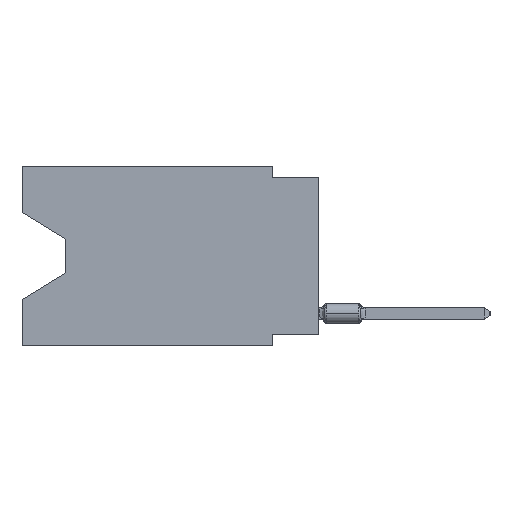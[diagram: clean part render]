
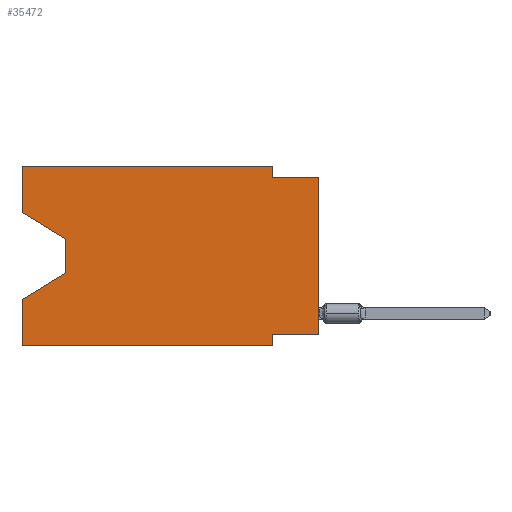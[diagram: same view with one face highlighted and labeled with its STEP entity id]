
A CAD part, left-side view. The second image highlights one B-rep face of the part: STEP entity #35472.
In plain terms, the highlighted planar face has unit normal (-1, 0, 0).
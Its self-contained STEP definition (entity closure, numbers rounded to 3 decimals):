
#967 = VERTEX_POINT ( 'NONE', #29241 ) ;
#978 = LINE ( 'NONE', #5575, #1717 ) ;
#1210 = CARTESIAN_POINT ( 'NONE',  ( 0., 0., -0.635 ) ) ;
#1267 = DIRECTION ( 'NONE',  ( 0., 0., 1. ) ) ;
#1576 = DIRECTION ( 'NONE',  ( 0., 0., 1. ) ) ;
#1717 = VECTOR ( 'NONE', #1576, 1000. ) ;
#2077 = VERTEX_POINT ( 'NONE', #21697 ) ;
#2115 = LINE ( 'NONE', #16244, #34366 ) ;
#3114 = EDGE_CURVE ( 'NONE', #31184, #11904, #978, .T. ) ;
#3126 = CARTESIAN_POINT ( 'NONE',  ( 0., 0., 0. ) ) ;
#5131 = EDGE_CURVE ( 'NONE', #29880, #53649, #2115, .T. ) ;
#5323 = EDGE_LOOP ( 'NONE', ( #9318, #32974, #53867, #51299, #5969, #42770, #48127, #58527, #47879, #10838, #58053, #54264 ) ) ;
#5575 = CARTESIAN_POINT ( 'NONE',  ( 0., 16.383, 0. ) ) ;
#5668 = VECTOR ( 'NONE', #20472, 1000. ) ;
#5870 = CARTESIAN_POINT ( 'NONE',  ( 0., 16.383, 0. ) ) ;
#5969 = ORIENTED_EDGE ( 'NONE', *, *, #59230, .T. ) ;
#6112 = PLANE ( 'NONE',  #14296 ) ;
#6342 = LINE ( 'NONE', #15268, #5668 ) ;
#6634 = CARTESIAN_POINT ( 'NONE',  ( 0., 16.383, -2.546 ) ) ;
#6934 = LINE ( 'NONE', #19030, #54746 ) ;
#7481 = LINE ( 'NONE', #58170, #37484 ) ;
#7900 = EDGE_CURVE ( 'NONE', #38194, #13895, #7481, .T. ) ;
#8309 = CARTESIAN_POINT ( 'NONE',  ( 0., 16.383, 0. ) ) ;
#9318 = ORIENTED_EDGE ( 'NONE', *, *, #32489, .T. ) ;
#9823 = DIRECTION ( 'NONE',  ( 0., 0., -1. ) ) ;
#10111 = DIRECTION ( 'NONE',  ( 0., 0., -1. ) ) ;
#10654 = LINE ( 'NONE', #14659, #21511 ) ;
#10771 = LINE ( 'NONE', #20596, #28127 ) ;
#10838 = ORIENTED_EDGE ( 'NONE', *, *, #7900, .F. ) ;
#11307 = CARTESIAN_POINT ( 'NONE',  ( 0., 13.97, -5.893 ) ) ;
#11727 = EDGE_CURVE ( 'NONE', #967, #2077, #53460, .T. ) ;
#11904 = VERTEX_POINT ( 'NONE', #8309 ) ;
#13895 = VERTEX_POINT ( 'NONE', #43415 ) ;
#14072 = VECTOR ( 'NONE', #20836, 1000. ) ;
#14296 = AXIS2_PLACEMENT_3D ( 'NONE', #24871, #57719, #9823 ) ;
#14659 = CARTESIAN_POINT ( 'NONE',  ( 0., 0., -9.271 ) ) ;
#15268 = CARTESIAN_POINT ( 'NONE',  ( 0., 16.383, 0. ) ) ;
#15713 = CARTESIAN_POINT ( 'NONE',  ( 0., 2.54, -9.906 ) ) ;
#15995 = DIRECTION ( 'NONE',  ( 0., -1., 0. ) ) ;
#16244 = CARTESIAN_POINT ( 'NONE',  ( 0., 2.54, -9.906 ) ) ;
#16991 = LINE ( 'NONE', #21292, #18967 ) ;
#18967 = VECTOR ( 'NONE', #20376, 1000. ) ;
#19030 = CARTESIAN_POINT ( 'NONE',  ( 0., 13.97, -4.013 ) ) ;
#19507 = DIRECTION ( 'NONE',  ( 0., -1., 0. ) ) ;
#20376 = DIRECTION ( 'NONE',  ( 0., -0.855, -0.519 ) ) ;
#20472 = DIRECTION ( 'NONE',  ( 0., -1., 0. ) ) ;
#20596 = CARTESIAN_POINT ( 'NONE',  ( 0., 0., -0.635 ) ) ;
#20694 = DIRECTION ( 'NONE',  ( 0., 0., -1. ) ) ;
#20836 = DIRECTION ( 'NONE',  ( 0., 0.855, -0.519 ) ) ;
#20848 = DIRECTION ( 'NONE',  ( 0., 0., -1. ) ) ;
#21292 = CARTESIAN_POINT ( 'NONE',  ( 0., 16.383, -2.546 ) ) ;
#21511 = VECTOR ( 'NONE', #52436, 1000. ) ;
#21697 = CARTESIAN_POINT ( 'NONE',  ( 0., 16.383, -7.36 ) ) ;
#24871 = CARTESIAN_POINT ( 'NONE',  ( 0., 16.383, 0. ) ) ;
#25377 = CARTESIAN_POINT ( 'NONE',  ( 0., 2.54, -9.271 ) ) ;
#25723 = EDGE_CURVE ( 'NONE', #29432, #28521, #31078, .T. ) ;
#27643 = CARTESIAN_POINT ( 'NONE',  ( 0., 2.54, 0. ) ) ;
#28127 = VECTOR ( 'NONE', #15995, 1000. ) ;
#28521 = VERTEX_POINT ( 'NONE', #1210 ) ;
#29241 = CARTESIAN_POINT ( 'NONE',  ( 0., 16.383, -9.906 ) ) ;
#29271 = VECTOR ( 'NONE', #1267, 1000. ) ;
#29432 = VERTEX_POINT ( 'NONE', #54472 ) ;
#29880 = VERTEX_POINT ( 'NONE', #25377 ) ;
#31078 = LINE ( 'NONE', #3126, #41121 ) ;
#31184 = VERTEX_POINT ( 'NONE', #6634 ) ;
#32489 = EDGE_CURVE ( 'NONE', #31184, #57374, #16991, .T. ) ;
#32732 = CARTESIAN_POINT ( 'NONE',  ( 0., 16.383, -9.906 ) ) ;
#32974 = ORIENTED_EDGE ( 'NONE', *, *, #47713, .T. ) ;
#34366 = VECTOR ( 'NONE', #20848, 1000. ) ;
#35442 = CARTESIAN_POINT ( 'NONE',  ( 0., 13.97, -5.893 ) ) ;
#35472 = ADVANCED_FACE ( 'NONE', ( #48188 ), #6112, .F. ) ;
#35502 = VECTOR ( 'NONE', #19507, 1000. ) ;
#37484 = VECTOR ( 'NONE', #20694, 1000. ) ;
#38194 = VERTEX_POINT ( 'NONE', #27643 ) ;
#40807 = EDGE_CURVE ( 'NONE', #53340, #2077, #53386, .T. ) ;
#40887 = DIRECTION ( 'NONE',  ( 0., 0., 1. ) ) ;
#41121 = VECTOR ( 'NONE', #40887, 1000. ) ;
#42770 = ORIENTED_EDGE ( 'NONE', *, *, #5131, .F. ) ;
#43415 = CARTESIAN_POINT ( 'NONE',  ( 0., 2.54, -0.635 ) ) ;
#44477 = EDGE_CURVE ( 'NONE', #13895, #28521, #10771, .T. ) ;
#47713 = EDGE_CURVE ( 'NONE', #57374, #53340, #6934, .T. ) ;
#47879 = ORIENTED_EDGE ( 'NONE', *, *, #44477, .F. ) ;
#48127 = ORIENTED_EDGE ( 'NONE', *, *, #55500, .F. ) ;
#48188 = FACE_OUTER_BOUND ( 'NONE', #5323, .T. ) ;
#51299 = ORIENTED_EDGE ( 'NONE', *, *, #11727, .F. ) ;
#52436 = DIRECTION ( 'NONE',  ( 0., 1., 0. ) ) ;
#53340 = VERTEX_POINT ( 'NONE', #35442 ) ;
#53386 = LINE ( 'NONE', #11307, #14072 ) ;
#53460 = LINE ( 'NONE', #5870, #29271 ) ;
#53649 = VERTEX_POINT ( 'NONE', #15713 ) ;
#53867 = ORIENTED_EDGE ( 'NONE', *, *, #40807, .T. ) ;
#53906 = EDGE_CURVE ( 'NONE', #11904, #38194, #6342, .T. ) ;
#54012 = CARTESIAN_POINT ( 'NONE',  ( 0., 13.97, -4.013 ) ) ;
#54264 = ORIENTED_EDGE ( 'NONE', *, *, #3114, .F. ) ;
#54472 = CARTESIAN_POINT ( 'NONE',  ( 0., 0., -9.271 ) ) ;
#54746 = VECTOR ( 'NONE', #10111, 1000. ) ;
#55500 = EDGE_CURVE ( 'NONE', #29432, #29880, #10654, .T. ) ;
#55762 = LINE ( 'NONE', #32732, #35502 ) ;
#57374 = VERTEX_POINT ( 'NONE', #54012 ) ;
#57719 = DIRECTION ( 'NONE',  ( 1., 0., 0. ) ) ;
#58053 = ORIENTED_EDGE ( 'NONE', *, *, #53906, .F. ) ;
#58170 = CARTESIAN_POINT ( 'NONE',  ( 0., 2.54, 0. ) ) ;
#58527 = ORIENTED_EDGE ( 'NONE', *, *, #25723, .T. ) ;
#59230 = EDGE_CURVE ( 'NONE', #967, #53649, #55762, .T. ) ;
